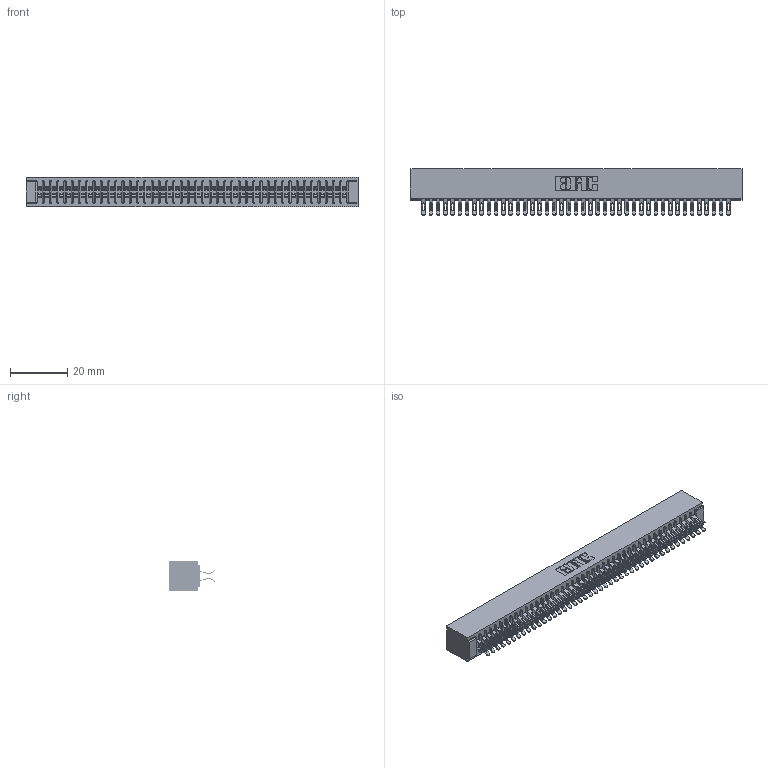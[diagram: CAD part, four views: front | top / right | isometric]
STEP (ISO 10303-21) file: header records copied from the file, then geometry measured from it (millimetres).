
FILE_DESCRIPTION (( 'STEP AP203' ), '1' );
FILE_NAME ('391-086-555-201.STEP', '2018-08-09T16:46:15', ( '' ), ( '' ), 'SwSTEP 2.0', 'SolidWorks 2016', '' );
FILE_SCHEMA (( 'CONFIG_CONTROL_DESIGN' ));
Length unit declared in the file: inch
Products named in the file (3): 391-086-555-201; 341 Part_No Mounting Lugs; 341-292-001_341-292-155
Assembly tree (87 placements, depth 2):
  391-086-555-201
    341 Part_No Mounting Lugs
    341-292-001_341-292-155  x86
Bounding box: 116.2 x 16.31 x 10.16 mm (x, y, z)
Volume: 8927.2 mm3; surface area: 17242.6 mm2
Topology: 87 solids, 87 shells, 6816 faces, 20373 edges, 13262 vertices
Faces by surface type: plane 3676, cylinder 2968, sphere 88, torus 84
Entity records: 52098 total; most frequent: CARTESIAN_POINT 8675, ORIENTED_EDGE 8610, DIRECTION 8407, EDGE_CURVE 4305, LINE 3467, VECTOR 3467, VERTEX_POINT 2722, AXIS2_PLACEMENT_3D 2470
